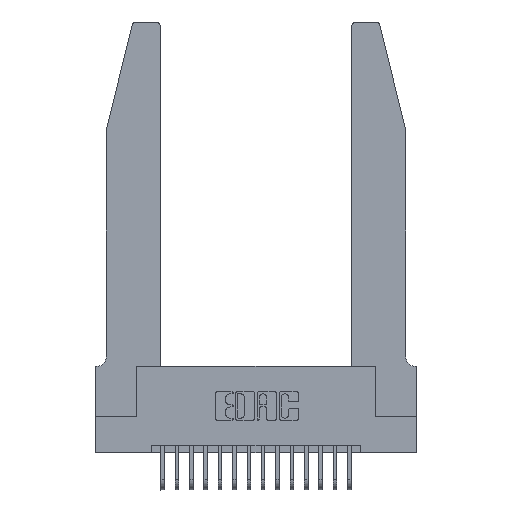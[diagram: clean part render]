
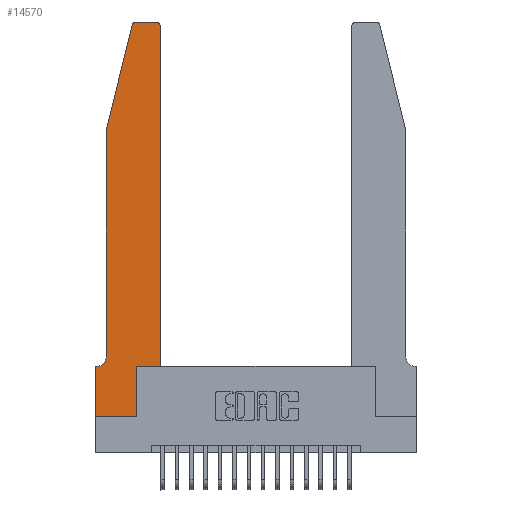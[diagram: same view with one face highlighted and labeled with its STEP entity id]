
A CAD part, top view. The second image highlights one B-rep face of the part: STEP entity #14570.
In plain terms, the highlighted planar face has unit normal (0, 0, 1).
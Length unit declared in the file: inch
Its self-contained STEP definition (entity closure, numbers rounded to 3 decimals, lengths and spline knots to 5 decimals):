
#13 = ORIENTED_EDGE ( 'NONE', *, *, #16571, .T. ) ;
#14 = CARTESIAN_POINT ( 'NONE',  ( 0.2865, 0.35, 0.37 ) ) ;
#169 = ORIENTED_EDGE ( 'NONE', *, *, #466, .T. ) ;
#408 = ORIENTED_EDGE ( 'NONE', *, *, #5817, .T. ) ;
#466 = EDGE_CURVE ( 'NONE', #18803, #2958, #5898, .T. ) ;
#747 = DIRECTION ( 'NONE',  ( 0., 0., 1. ) ) ;
#772 = CARTESIAN_POINT ( 'NONE',  ( 0.2605, 2.75, 0.37 ) ) ;
#961 = LINE ( 'NONE', #7804, #8459 ) ;
#1855 = CARTESIAN_POINT ( 'NONE',  ( 0.2865, 0., 0.37 ) ) ;
#2445 = ORIENTED_EDGE ( 'NONE', *, *, #7200, .T. ) ;
#2600 = AXIS2_PLACEMENT_3D ( 'NONE', #14025, #747, #11143 ) ;
#2623 = ORIENTED_EDGE ( 'NONE', *, *, #11023, .T. ) ;
#2706 = VERTEX_POINT ( 'NONE', #9463 ) ;
#2792 = DIRECTION ( 'NONE',  ( -0.239, -0.971, 0. ) ) ;
#2862 = ORIENTED_EDGE ( 'NONE', *, *, #6768, .T. ) ;
#2958 = VERTEX_POINT ( 'NONE', #15873 ) ;
#3173 = CARTESIAN_POINT ( 'NONE',  ( 0., 0., 0.37 ) ) ;
#3458 = CARTESIAN_POINT ( 'NONE',  ( 0.4505, 0.35, 0.37 ) ) ;
#3493 = ORIENTED_EDGE ( 'NONE', *, *, #12506, .T. ) ;
#3741 = CARTESIAN_POINT ( 'NONE',  ( 0.0755, 2., 0.37 ) ) ;
#3777 = DIRECTION ( 'NONE',  ( -1., 0., 0. ) ) ;
#3799 = ORIENTED_EDGE ( 'NONE', *, *, #4601, .T. ) ;
#4088 = DIRECTION ( 'NONE',  ( 0., -1., 0. ) ) ;
#4249 = ORIENTED_EDGE ( 'NONE', *, *, #12368, .T. ) ;
#4601 = EDGE_CURVE ( 'NONE', #2706, #7764, #18558, .T. ) ;
#5157 = CARTESIAN_POINT ( 'NONE',  ( 0.4505, 0.35, 0.37 ) ) ;
#5432 = CARTESIAN_POINT ( 'NONE',  ( 0.2865, 0.35, 0.37 ) ) ;
#5543 = LINE ( 'NONE', #5432, #9052 ) ;
#5817 = EDGE_CURVE ( 'NONE', #2958, #15749, #6601, .T. ) ;
#5830 = DIRECTION ( 'NONE',  ( 1., 0., 0. ) ) ;
#5898 = LINE ( 'NONE', #14475, #6094 ) ;
#6089 = LINE ( 'NONE', #10101, #9586 ) ;
#6094 = VECTOR ( 'NONE', #17337, 39.37008 ) ;
#6266 = CARTESIAN_POINT ( 'NONE',  ( 0.4205, 2.72, 0.37 ) ) ;
#6346 = ORIENTED_EDGE ( 'NONE', *, *, #17921, .T. ) ;
#6431 = VERTEX_POINT ( 'NONE', #16296 ) ;
#6601 = CIRCLE ( 'NONE', #14618, 0.03 ) ;
#6768 = EDGE_CURVE ( 'NONE', #14397, #18131, #10759, .T. ) ;
#6893 = EDGE_LOOP ( 'NONE', ( #2445, #2623, #6346, #10788, #4249, #3799, #3493, #2862, #9211, #13, #169, #408 ) ) ;
#6940 = DIRECTION ( 'NONE',  ( 0., 1., 0. ) ) ;
#7200 = EDGE_CURVE ( 'NONE', #15749, #13133, #15530, .T. ) ;
#7239 = CARTESIAN_POINT ( 'NONE',  ( 0.0755, 2., 0.37 ) ) ;
#7248 = DIRECTION ( 'NONE',  ( 0., 0., 1. ) ) ;
#7745 = DIRECTION ( 'NONE',  ( -1., 0., 0. ) ) ;
#7764 = VERTEX_POINT ( 'NONE', #7900 ) ;
#7768 = DIRECTION ( 'NONE',  ( 1., 0., 0. ) ) ;
#7804 = CARTESIAN_POINT ( 'NONE',  ( 0.0755, 2., 0.37 ) ) ;
#7900 = CARTESIAN_POINT ( 'NONE',  ( 0., 0.35, 0.37 ) ) ;
#8301 = DIRECTION ( 'NONE',  ( 0., 0., -1. ) ) ;
#8434 = CIRCLE ( 'NONE', #16388, 0.07 ) ;
#8459 = VECTOR ( 'NONE', #9295, 39.37008 ) ;
#9052 = VECTOR ( 'NONE', #6940, 39.37008 ) ;
#9067 = FACE_OUTER_BOUND ( 'NONE', #6893, .T. ) ;
#9211 = ORIENTED_EDGE ( 'NONE', *, *, #15045, .T. ) ;
#9295 = DIRECTION ( 'NONE',  ( 0., -1., 0. ) ) ;
#9463 = CARTESIAN_POINT ( 'NONE',  ( 0.0055, 0.35, 0.37 ) ) ;
#9534 = VECTOR ( 'NONE', #18214, 39.37008 ) ;
#9586 = VECTOR ( 'NONE', #4088, 39.37008 ) ;
#10101 = CARTESIAN_POINT ( 'NONE',  ( 0., 0., 0.37 ) ) ;
#10390 = VECTOR ( 'NONE', #2792, 39.37008 ) ;
#10759 = LINE ( 'NONE', #14638, #18516 ) ;
#10788 = ORIENTED_EDGE ( 'NONE', *, *, #11886, .T. ) ;
#11023 = EDGE_CURVE ( 'NONE', #13133, #12253, #11910, .T. ) ;
#11136 = VERTEX_POINT ( 'NONE', #14 ) ;
#11143 = DIRECTION ( 'NONE',  ( 1., 0., 0. ) ) ;
#11249 = VECTOR ( 'NONE', #7745, 39.37008 ) ;
#11886 = EDGE_CURVE ( 'NONE', #13001, #6431, #961, .T. ) ;
#11910 = CIRCLE ( 'NONE', #15898, 0.03 ) ;
#12253 = VERTEX_POINT ( 'NONE', #12972 ) ;
#12368 = EDGE_CURVE ( 'NONE', #6431, #2706, #8434, .T. ) ;
#12506 = EDGE_CURVE ( 'NONE', #7764, #14397, #6089, .T. ) ;
#12972 = CARTESIAN_POINT ( 'NONE',  ( 0.25487, 2.72718, 0.37 ) ) ;
#13001 = VERTEX_POINT ( 'NONE', #3741 ) ;
#13133 = VERTEX_POINT ( 'NONE', #17316 ) ;
#14025 = CARTESIAN_POINT ( 'NONE',  ( 0., 0.35, 0.37 ) ) ;
#14257 = LINE ( 'NONE', #7239, #10390 ) ;
#14397 = VERTEX_POINT ( 'NONE', #3173 ) ;
#14475 = CARTESIAN_POINT ( 'NONE',  ( 0.4505, 0.35, 0.37 ) ) ;
#14570 = ADVANCED_FACE ( 'NONE', ( #9067 ), #15488, .T. ) ;
#14618 = AXIS2_PLACEMENT_3D ( 'NONE', #6266, #16505, #7768 ) ;
#14638 = CARTESIAN_POINT ( 'NONE',  ( 0., 0., 0.37 ) ) ;
#15045 = EDGE_CURVE ( 'NONE', #18131, #11136, #5543, .T. ) ;
#15488 = PLANE ( 'NONE',  #2600 ) ;
#15530 = LINE ( 'NONE', #772, #18959 ) ;
#15749 = VERTEX_POINT ( 'NONE', #17342 ) ;
#15873 = CARTESIAN_POINT ( 'NONE',  ( 0.4505, 2.72, 0.37 ) ) ;
#15898 = AXIS2_PLACEMENT_3D ( 'NONE', #16010, #7248, #17473 ) ;
#16010 = CARTESIAN_POINT ( 'NONE',  ( 0.284, 2.72, 0.37 ) ) ;
#16296 = CARTESIAN_POINT ( 'NONE',  ( 0.0755, 0.42, 0.37 ) ) ;
#16388 = AXIS2_PLACEMENT_3D ( 'NONE', #17028, #8301, #18508 ) ;
#16490 = CARTESIAN_POINT ( 'NONE',  ( 0.0755, 0.35, 0.37 ) ) ;
#16505 = DIRECTION ( 'NONE',  ( 0., 0., 1. ) ) ;
#16571 = EDGE_CURVE ( 'NONE', #11136, #18803, #17730, .T. ) ;
#17028 = CARTESIAN_POINT ( 'NONE',  ( 0.0055, 0.42, 0.37 ) ) ;
#17316 = CARTESIAN_POINT ( 'NONE',  ( 0.284, 2.75, 0.37 ) ) ;
#17337 = DIRECTION ( 'NONE',  ( 0., 1., 0. ) ) ;
#17342 = CARTESIAN_POINT ( 'NONE',  ( 0.4205, 2.75, 0.37 ) ) ;
#17473 = DIRECTION ( 'NONE',  ( 1., 0., 0. ) ) ;
#17730 = LINE ( 'NONE', #3458, #9534 ) ;
#17921 = EDGE_CURVE ( 'NONE', #12253, #13001, #14257, .T. ) ;
#18131 = VERTEX_POINT ( 'NONE', #1855 ) ;
#18214 = DIRECTION ( 'NONE',  ( 1., 0., 0. ) ) ;
#18508 = DIRECTION ( 'NONE',  ( -1., 0., 0. ) ) ;
#18516 = VECTOR ( 'NONE', #5830, 39.37008 ) ;
#18558 = LINE ( 'NONE', #16490, #11249 ) ;
#18803 = VERTEX_POINT ( 'NONE', #5157 ) ;
#18959 = VECTOR ( 'NONE', #3777, 39.37008 ) ;
